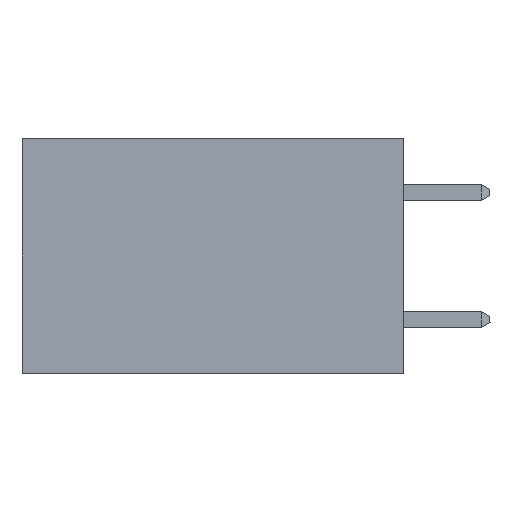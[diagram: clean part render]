
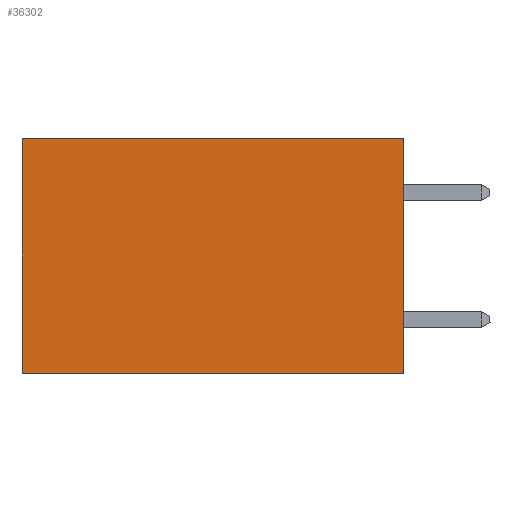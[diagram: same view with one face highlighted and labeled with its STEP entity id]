
A CAD part, left-side view. The second image highlights one B-rep face of the part: STEP entity #36302.
In plain terms, the highlighted planar face has unit normal (-1, 0, 0).
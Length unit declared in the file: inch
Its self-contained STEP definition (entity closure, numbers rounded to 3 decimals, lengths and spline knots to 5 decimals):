
#658 = DIRECTION ( 'NONE',  ( 0., 1., 0. ) ) ;
#1994 = VERTEX_POINT ( 'NONE', #38400 ) ;
#2567 = VERTEX_POINT ( 'NONE', #5792 ) ;
#2894 = LINE ( 'NONE', #17322, #11287 ) ;
#3779 = LINE ( 'NONE', #10104, #27986 ) ;
#5505 = CARTESIAN_POINT ( 'NONE',  ( 0.2875, 0.6, 0. ) ) ;
#5792 = CARTESIAN_POINT ( 'NONE',  ( 0.2875, 0., 0. ) ) ;
#6288 = VERTEX_POINT ( 'NONE', #13508 ) ;
#7748 = EDGE_CURVE ( 'NONE', #2567, #1994, #2894, .T. ) ;
#8654 = DIRECTION ( 'NONE',  ( 0., 0., -1. ) ) ;
#8857 = CARTESIAN_POINT ( 'NONE',  ( 0.2875, 0., 0. ) ) ;
#10104 = CARTESIAN_POINT ( 'NONE',  ( 0.2875, 0., -0.37 ) ) ;
#10226 = VECTOR ( 'NONE', #31182, 39.37008 ) ;
#11287 = VECTOR ( 'NONE', #32950, 39.37008 ) ;
#12078 = DIRECTION ( 'NONE',  ( 0., 0., -1. ) ) ;
#13508 = CARTESIAN_POINT ( 'NONE',  ( 0.2875, 0., -0.37 ) ) ;
#16417 = AXIS2_PLACEMENT_3D ( 'NONE', #8857, #30915, #12078 ) ;
#17322 = CARTESIAN_POINT ( 'NONE',  ( 0.2875, 0., 0. ) ) ;
#18291 = PLANE ( 'NONE',  #16417 ) ;
#18725 = ORIENTED_EDGE ( 'NONE', *, *, #30885, .F. ) ;
#19658 = FACE_OUTER_BOUND ( 'NONE', #24958, .T. ) ;
#22107 = ORIENTED_EDGE ( 'NONE', *, *, #33020, .T. ) ;
#22379 = VECTOR ( 'NONE', #8654, 39.37008 ) ;
#24958 = EDGE_LOOP ( 'NONE', ( #22107, #18725, #38386, #39047 ) ) ;
#27067 = LINE ( 'NONE', #37215, #10226 ) ;
#27986 = VECTOR ( 'NONE', #658, 39.37008 ) ;
#29880 = CARTESIAN_POINT ( 'NONE',  ( 0.2875, 0.6, -0.37 ) ) ;
#30885 = EDGE_CURVE ( 'NONE', #6288, #33531, #3779, .T. ) ;
#30915 = DIRECTION ( 'NONE',  ( 1., 0., 0. ) ) ;
#31182 = DIRECTION ( 'NONE',  ( 0., 0., -1. ) ) ;
#32950 = DIRECTION ( 'NONE',  ( 0., 1., 0. ) ) ;
#33020 = EDGE_CURVE ( 'NONE', #1994, #33531, #38876, .T. ) ;
#33531 = VERTEX_POINT ( 'NONE', #29880 ) ;
#36302 = ADVANCED_FACE ( 'NONE', ( #19658 ), #18291, .F. ) ;
#36355 = EDGE_CURVE ( 'NONE', #2567, #6288, #27067, .T. ) ;
#37215 = CARTESIAN_POINT ( 'NONE',  ( 0.2875, 0., 0. ) ) ;
#38386 = ORIENTED_EDGE ( 'NONE', *, *, #36355, .F. ) ;
#38400 = CARTESIAN_POINT ( 'NONE',  ( 0.2875, 0.6, 0. ) ) ;
#38876 = LINE ( 'NONE', #5505, #22379 ) ;
#39047 = ORIENTED_EDGE ( 'NONE', *, *, #7748, .T. ) ;
